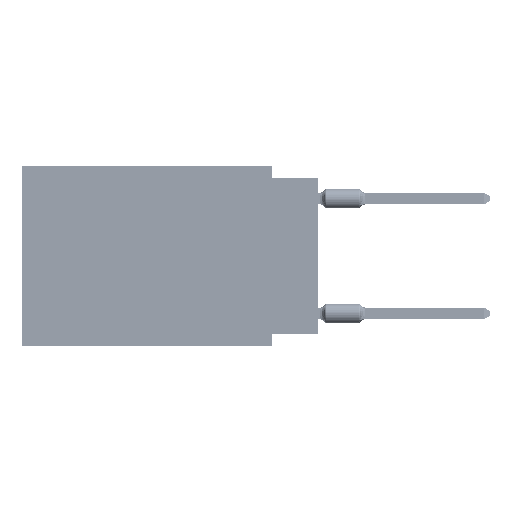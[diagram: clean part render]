
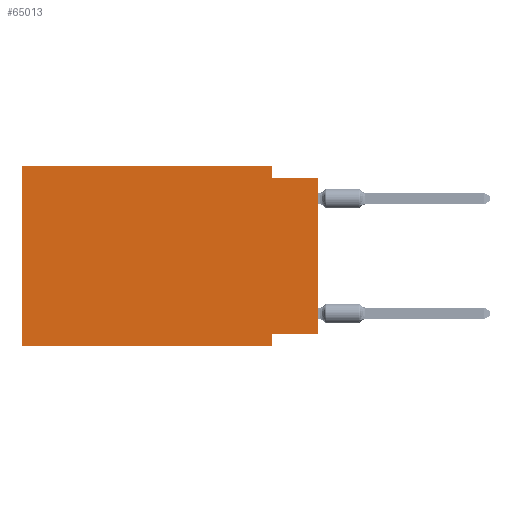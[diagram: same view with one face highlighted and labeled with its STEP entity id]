
A CAD part, left-side view. The second image highlights one B-rep face of the part: STEP entity #65013.
In plain terms, the highlighted planar face has unit normal (-1, 0, 0).
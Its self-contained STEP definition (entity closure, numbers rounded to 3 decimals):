
#1799 = DIRECTION ( 'NONE',  ( 1., 0., 0. ) ) ;
#2085 = VECTOR ( 'NONE', #74139, 1000. ) ;
#2839 = LINE ( 'NONE', #35020, #59790 ) ;
#2976 = ORIENTED_EDGE ( 'NONE', *, *, #57381, .F. ) ;
#3786 = LINE ( 'NONE', #69978, #68238 ) ;
#4752 = CARTESIAN_POINT ( 'NONE',  ( 0., 16.383, 0. ) ) ;
#6849 = EDGE_CURVE ( 'NONE', #49027, #12481, #49816, .T. ) ;
#8968 = DIRECTION ( 'NONE',  ( 0., 0., -1. ) ) ;
#9736 = EDGE_CURVE ( 'NONE', #32412, #18427, #77269, .T. ) ;
#10559 = CARTESIAN_POINT ( 'NONE',  ( 0., 2.54, 0. ) ) ;
#12159 = CARTESIAN_POINT ( 'NONE',  ( 0., 2.54, -0.635 ) ) ;
#12331 = CARTESIAN_POINT ( 'NONE',  ( 0., 0., 0. ) ) ;
#12481 = VERTEX_POINT ( 'NONE', #16557 ) ;
#15162 = AXIS2_PLACEMENT_3D ( 'NONE', #26517, #1799, #8968 ) ;
#16307 = ORIENTED_EDGE ( 'NONE', *, *, #20651, .F. ) ;
#16557 = CARTESIAN_POINT ( 'NONE',  ( 0., 0., -0.635 ) ) ;
#18427 = VERTEX_POINT ( 'NONE', #27152 ) ;
#20108 = FACE_OUTER_BOUND ( 'NONE', #72564, .T. ) ;
#20530 = LINE ( 'NONE', #56471, #52892 ) ;
#20651 = EDGE_CURVE ( 'NONE', #66425, #12481, #37594, .T. ) ;
#21383 = ORIENTED_EDGE ( 'NONE', *, *, #77350, .F. ) ;
#21771 = VERTEX_POINT ( 'NONE', #10559 ) ;
#22212 = CARTESIAN_POINT ( 'NONE',  ( 0., 2.54, -9.906 ) ) ;
#25749 = DIRECTION ( 'NONE',  ( 0., 0., -1. ) ) ;
#26517 = CARTESIAN_POINT ( 'NONE',  ( 0., 16.383, 0. ) ) ;
#26832 = ORIENTED_EDGE ( 'NONE', *, *, #32599, .F. ) ;
#27152 = CARTESIAN_POINT ( 'NONE',  ( 0., 2.54, -9.906 ) ) ;
#27196 = CARTESIAN_POINT ( 'NONE',  ( 0., 16.383, -9.906 ) ) ;
#28105 = VECTOR ( 'NONE', #70487, 1000. ) ;
#29084 = DIRECTION ( 'NONE',  ( 0., -1., 0. ) ) ;
#29145 = ORIENTED_EDGE ( 'NONE', *, *, #29927, .F. ) ;
#29927 = EDGE_CURVE ( 'NONE', #21771, #66425, #20530, .T. ) ;
#32320 = ORIENTED_EDGE ( 'NONE', *, *, #38575, .T. ) ;
#32412 = VERTEX_POINT ( 'NONE', #55261 ) ;
#32599 = EDGE_CURVE ( 'NONE', #49027, #32412, #3786, .T. ) ;
#35020 = CARTESIAN_POINT ( 'NONE',  ( 0., 16.383, -9.906 ) ) ;
#37594 = LINE ( 'NONE', #67534, #52488 ) ;
#38575 = EDGE_CURVE ( 'NONE', #50365, #18427, #2839, .T. ) ;
#39258 = DIRECTION ( 'NONE',  ( 0., 1., 0. ) ) ;
#41593 = CARTESIAN_POINT ( 'NONE',  ( 0., 16.383, 0. ) ) ;
#41633 = DIRECTION ( 'NONE',  ( 0., 0., 1. ) ) ;
#42808 = CARTESIAN_POINT ( 'NONE',  ( 0., 16.383, 0. ) ) ;
#43962 = DIRECTION ( 'NONE',  ( 0., -1., 0. ) ) ;
#44311 = CARTESIAN_POINT ( 'NONE',  ( 0., 0., -9.271 ) ) ;
#44924 = VECTOR ( 'NONE', #29084, 1000. ) ;
#49027 = VERTEX_POINT ( 'NONE', #44311 ) ;
#49816 = LINE ( 'NONE', #12331, #2085 ) ;
#50365 = VERTEX_POINT ( 'NONE', #27196 ) ;
#52488 = VECTOR ( 'NONE', #43962, 1000. ) ;
#52884 = ORIENTED_EDGE ( 'NONE', *, *, #6849, .T. ) ;
#52892 = VECTOR ( 'NONE', #25749, 1000. ) ;
#53737 = DIRECTION ( 'NONE',  ( 0., -1., 0. ) ) ;
#55261 = CARTESIAN_POINT ( 'NONE',  ( 0., 2.54, -9.271 ) ) ;
#56471 = CARTESIAN_POINT ( 'NONE',  ( 0., 2.54, 0. ) ) ;
#57381 = EDGE_CURVE ( 'NONE', #50365, #68546, #72349, .T. ) ;
#59398 = LINE ( 'NONE', #4752, #44924 ) ;
#59790 = VECTOR ( 'NONE', #53737, 1000. ) ;
#65013 = ADVANCED_FACE ( 'NONE', ( #20108 ), #75969, .F. ) ;
#66425 = VERTEX_POINT ( 'NONE', #12159 ) ;
#67534 = CARTESIAN_POINT ( 'NONE',  ( 0., 0., -0.635 ) ) ;
#68238 = VECTOR ( 'NONE', #39258, 1000. ) ;
#68546 = VERTEX_POINT ( 'NONE', #41593 ) ;
#69978 = CARTESIAN_POINT ( 'NONE',  ( 0., 0., -9.271 ) ) ;
#70487 = DIRECTION ( 'NONE',  ( 0., 0., -1. ) ) ;
#72349 = LINE ( 'NONE', #42808, #77037 ) ;
#72564 = EDGE_LOOP ( 'NONE', ( #52884, #16307, #29145, #21383, #2976, #32320, #77663, #26832 ) ) ;
#74139 = DIRECTION ( 'NONE',  ( 0., 0., 1. ) ) ;
#75969 = PLANE ( 'NONE',  #15162 ) ;
#77037 = VECTOR ( 'NONE', #41633, 1000. ) ;
#77269 = LINE ( 'NONE', #22212, #28105 ) ;
#77350 = EDGE_CURVE ( 'NONE', #68546, #21771, #59398, .T. ) ;
#77663 = ORIENTED_EDGE ( 'NONE', *, *, #9736, .F. ) ;
